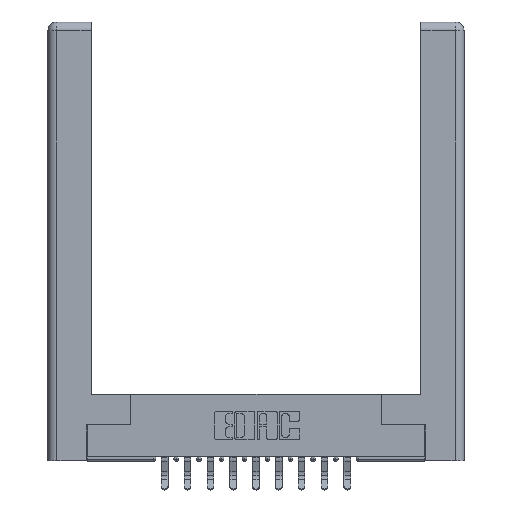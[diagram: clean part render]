
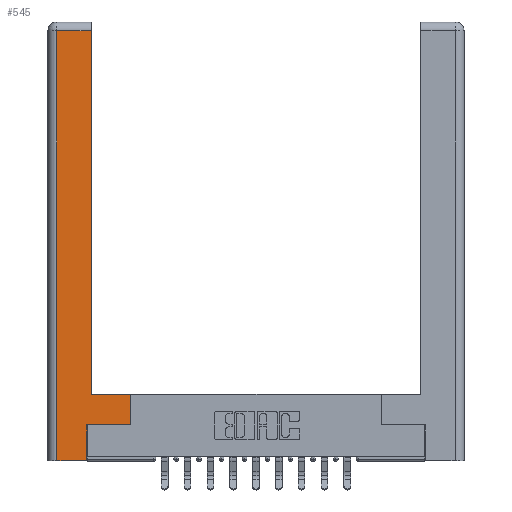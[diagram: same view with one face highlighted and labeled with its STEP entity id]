
A CAD part, top view. The second image highlights one B-rep face of the part: STEP entity #545.
In plain terms, the highlighted planar face has unit normal (0, 0, 1).
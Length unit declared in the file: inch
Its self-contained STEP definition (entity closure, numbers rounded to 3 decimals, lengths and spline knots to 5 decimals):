
#545 = ADVANCED_FACE ( 'NONE', ( #7156 ), #12072, .F. ) ;
#882 = CARTESIAN_POINT ( 'NONE',  ( 0.0615, 2.94, 0. ) ) ;
#1305 = EDGE_CURVE ( 'NONE', #8260, #10566, #12328, .T. ) ;
#1553 = VECTOR ( 'NONE', #10238, 39.37008 ) ;
#1805 = CARTESIAN_POINT ( 'NONE',  ( 0.0615, 0., 0. ) ) ;
#1910 = DIRECTION ( 'NONE',  ( -1., 0., 0. ) ) ;
#2032 = CARTESIAN_POINT ( 'NONE',  ( 0.0615, 2.94, 0. ) ) ;
#2400 = ORIENTED_EDGE ( 'NONE', *, *, #1305, .T. ) ;
#2459 = VERTEX_POINT ( 'NONE', #3772 ) ;
#2660 = VERTEX_POINT ( 'NONE', #7860 ) ;
#2950 = AXIS2_PLACEMENT_3D ( 'NONE', #14641, #9623, #1910 ) ;
#3301 = ORIENTED_EDGE ( 'NONE', *, *, #12087, .T. ) ;
#3486 = DIRECTION ( 'NONE',  ( -1., 0., 0. ) ) ;
#3772 = CARTESIAN_POINT ( 'NONE',  ( 0.565, 0.245, 0. ) ) ;
#3804 = DIRECTION ( 'NONE',  ( 0., 1., 0. ) ) ;
#4235 = EDGE_CURVE ( 'NONE', #2459, #8260, #9303, .T. ) ;
#4773 = LINE ( 'NONE', #12822, #10786 ) ;
#5263 = CARTESIAN_POINT ( 'NONE',  ( 0.0615, 0., 0. ) ) ;
#5371 = CARTESIAN_POINT ( 'NONE',  ( 0.265, 0., 0. ) ) ;
#5430 = EDGE_CURVE ( 'NONE', #2660, #12521, #11656, .T. ) ;
#5539 = CARTESIAN_POINT ( 'NONE',  ( 0.295, 0.45, 0. ) ) ;
#5983 = ORIENTED_EDGE ( 'NONE', *, *, #5430, .T. ) ;
#6262 = VECTOR ( 'NONE', #15850, 39.37008 ) ;
#7025 = VECTOR ( 'NONE', #15294, 39.37008 ) ;
#7156 = FACE_OUTER_BOUND ( 'NONE', #12856, .T. ) ;
#7368 = LINE ( 'NONE', #5371, #13960 ) ;
#7630 = CARTESIAN_POINT ( 'NONE',  ( 0.565, 0.45, 0. ) ) ;
#7845 = ORIENTED_EDGE ( 'NONE', *, *, #16157, .T. ) ;
#7860 = CARTESIAN_POINT ( 'NONE',  ( 0.295, 2.94, 0. ) ) ;
#8012 = VERTEX_POINT ( 'NONE', #12127 ) ;
#8260 = VERTEX_POINT ( 'NONE', #7630 ) ;
#8270 = DIRECTION ( 'NONE',  ( -1., 0., 0. ) ) ;
#8423 = ORIENTED_EDGE ( 'NONE', *, *, #9580, .T. ) ;
#8877 = LINE ( 'NONE', #1805, #6262 ) ;
#9180 = CARTESIAN_POINT ( 'NONE',  ( 0.565, 0.45, 0. ) ) ;
#9303 = LINE ( 'NONE', #9180, #10686 ) ;
#9580 = EDGE_CURVE ( 'NONE', #16155, #8012, #11634, .T. ) ;
#9623 = DIRECTION ( 'NONE',  ( 0., 0., -1. ) ) ;
#9752 = VECTOR ( 'NONE', #8270, 39.37008 ) ;
#9811 = LINE ( 'NONE', #13922, #1553 ) ;
#10158 = CARTESIAN_POINT ( 'NONE',  ( 0.265, 0.245, 0. ) ) ;
#10238 = DIRECTION ( 'NONE',  ( 1., 0., 0. ) ) ;
#10259 = EDGE_CURVE ( 'NONE', #8012, #2459, #9811, .T. ) ;
#10320 = VERTEX_POINT ( 'NONE', #5263 ) ;
#10403 = DIRECTION ( 'NONE',  ( 1., 0., 0. ) ) ;
#10566 = VERTEX_POINT ( 'NONE', #14355 ) ;
#10686 = VECTOR ( 'NONE', #11742, 39.37008 ) ;
#10786 = VECTOR ( 'NONE', #3804, 39.37008 ) ;
#11634 = LINE ( 'NONE', #10158, #7025 ) ;
#11656 = LINE ( 'NONE', #882, #15462 ) ;
#11742 = DIRECTION ( 'NONE',  ( 0., 1., 0. ) ) ;
#12072 = PLANE ( 'NONE',  #2950 ) ;
#12087 = EDGE_CURVE ( 'NONE', #10566, #2660, #4773, .T. ) ;
#12090 = CARTESIAN_POINT ( 'NONE',  ( 0.265, 0., 0. ) ) ;
#12127 = CARTESIAN_POINT ( 'NONE',  ( 0.265, 0.245, 0. ) ) ;
#12328 = LINE ( 'NONE', #5539, #9752 ) ;
#12521 = VERTEX_POINT ( 'NONE', #2032 ) ;
#12683 = ORIENTED_EDGE ( 'NONE', *, *, #12747, .T. ) ;
#12747 = EDGE_CURVE ( 'NONE', #10320, #16155, #7368, .T. ) ;
#12822 = CARTESIAN_POINT ( 'NONE',  ( 0.295, 3., 0. ) ) ;
#12856 = EDGE_LOOP ( 'NONE', ( #3301, #5983, #7845, #12683, #8423, #13446, #13911, #2400 ) ) ;
#13446 = ORIENTED_EDGE ( 'NONE', *, *, #10259, .T. ) ;
#13911 = ORIENTED_EDGE ( 'NONE', *, *, #4235, .T. ) ;
#13922 = CARTESIAN_POINT ( 'NONE',  ( 0.565, 0.245, 0. ) ) ;
#13960 = VECTOR ( 'NONE', #10403, 39.37008 ) ;
#14355 = CARTESIAN_POINT ( 'NONE',  ( 0.295, 0.45, 0. ) ) ;
#14641 = CARTESIAN_POINT ( 'NONE',  ( 0., 0., 0. ) ) ;
#15294 = DIRECTION ( 'NONE',  ( 0., 1., 0. ) ) ;
#15462 = VECTOR ( 'NONE', #3486, 39.37008 ) ;
#15850 = DIRECTION ( 'NONE',  ( 0., -1., 0. ) ) ;
#16155 = VERTEX_POINT ( 'NONE', #12090 ) ;
#16157 = EDGE_CURVE ( 'NONE', #12521, #10320, #8877, .T. ) ;
